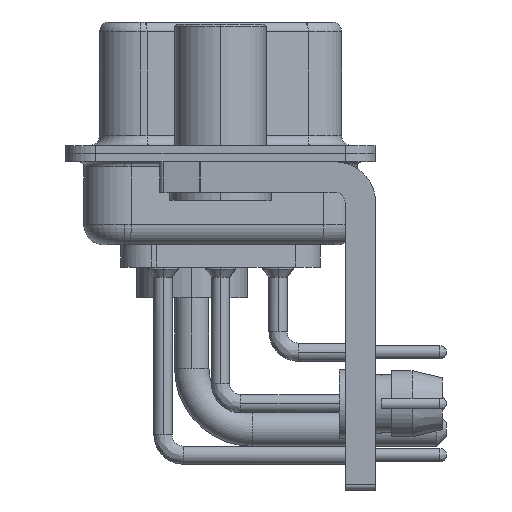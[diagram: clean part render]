
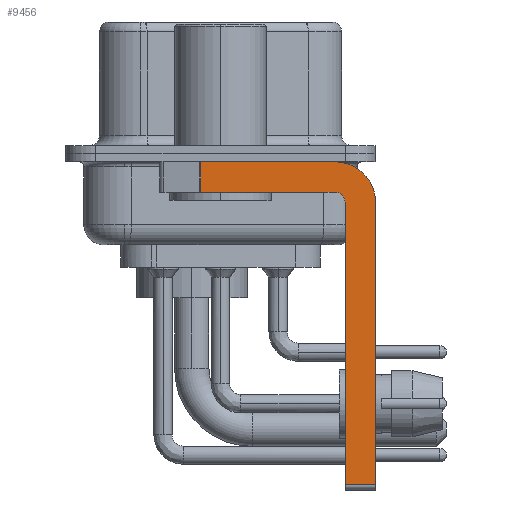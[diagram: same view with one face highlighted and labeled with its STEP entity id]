
A CAD part, left-side view. The second image highlights one B-rep face of the part: STEP entity #9456.
In plain terms, the highlighted planar face has unit normal (-1, 0, 0).
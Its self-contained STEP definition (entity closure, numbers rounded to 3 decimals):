
#649 = LINE ( 'NONE', #10176, #8430 ) ;
#1288 = VECTOR ( 'NONE', #22207, 1000. ) ;
#1503 = CARTESIAN_POINT ( 'NONE',  ( -2.9, -5.65, -2.4 ) ) ;
#1557 = DIRECTION ( 'NONE',  ( 0., 1., 0. ) ) ;
#1679 = CARTESIAN_POINT ( 'NONE',  ( -2.9, -5.65, -0.4 ) ) ;
#4796 = CARTESIAN_POINT ( 'NONE',  ( -2.9, -5.65, -2.4 ) ) ;
#5149 = ORIENTED_EDGE ( 'NONE', *, *, #18182, .T. ) ;
#5592 = EDGE_CURVE ( 'NONE', #38702, #24365, #30042, .T. ) ;
#5847 = CARTESIAN_POINT ( 'NONE',  ( -2.9, 0.978, -0.4 ) ) ;
#6621 = CARTESIAN_POINT ( 'NONE',  ( -2.9, -5.65, -2.4 ) ) ;
#6799 = DIRECTION ( 'NONE',  ( 0., -1., 0. ) ) ;
#8084 = DIRECTION ( 'NONE',  ( 0., -1., 0. ) ) ;
#8430 = VECTOR ( 'NONE', #22807, 1000. ) ;
#9301 = VERTEX_POINT ( 'NONE', #25941 ) ;
#9351 = VERTEX_POINT ( 'NONE', #12679 ) ;
#9456 = ADVANCED_FACE ( 'NONE', ( #14325 ), #29455, .F. ) ;
#9795 = AXIS2_PLACEMENT_3D ( 'NONE', #6621, #37888, #15529 ) ;
#10176 = CARTESIAN_POINT ( 'NONE',  ( -2.9, -7.65, -2.4 ) ) ;
#10959 = ORIENTED_EDGE ( 'NONE', *, *, #39089, .F. ) ;
#11698 = VECTOR ( 'NONE', #1557, 1000. ) ;
#12417 = ORIENTED_EDGE ( 'NONE', *, *, #38872, .T. ) ;
#12679 = CARTESIAN_POINT ( 'NONE',  ( -2.9, -6.15, -2.4 ) ) ;
#12680 = CARTESIAN_POINT ( 'NONE',  ( -2.9, 0.978, -1.9 ) ) ;
#12771 = AXIS2_PLACEMENT_3D ( 'NONE', #1503, #17257, #29246 ) ;
#14325 = FACE_OUTER_BOUND ( 'NONE', #33681, .T. ) ;
#15198 = AXIS2_PLACEMENT_3D ( 'NONE', #4796, #23451, #36061 ) ;
#15529 = DIRECTION ( 'NONE',  ( 0., 0., 1. ) ) ;
#16122 = LINE ( 'NONE', #28753, #18480 ) ;
#16672 = CARTESIAN_POINT ( 'NONE',  ( -2.9, -5.65, -1.9 ) ) ;
#17257 = DIRECTION ( 'NONE',  ( 1., 0., 0. ) ) ;
#17789 = ORIENTED_EDGE ( 'NONE', *, *, #5592, .F. ) ;
#18182 = EDGE_CURVE ( 'NONE', #24599, #9301, #16122, .T. ) ;
#18466 = CARTESIAN_POINT ( 'NONE',  ( -2.9, -6.15, -16.6 ) ) ;
#18480 = VECTOR ( 'NONE', #6799, 1000. ) ;
#19978 = LINE ( 'NONE', #16672, #11698 ) ;
#20207 = EDGE_CURVE ( 'NONE', #28423, #9301, #649, .T. ) ;
#20610 = EDGE_CURVE ( 'NONE', #9351, #23227, #26328, .T. ) ;
#21764 = LINE ( 'NONE', #18466, #39908 ) ;
#22207 = DIRECTION ( 'NONE',  ( 0., 0., -1. ) ) ;
#22807 = DIRECTION ( 'NONE',  ( 0., 0., -1. ) ) ;
#23227 = VERTEX_POINT ( 'NONE', #28762 ) ;
#23451 = DIRECTION ( 'NONE',  ( 1., 0., 0. ) ) ;
#24365 = VERTEX_POINT ( 'NONE', #1679 ) ;
#24599 = VERTEX_POINT ( 'NONE', #40765 ) ;
#25451 = ORIENTED_EDGE ( 'NONE', *, *, #35139, .F. ) ;
#25941 = CARTESIAN_POINT ( 'NONE',  ( -2.9, -7.65, -16.35 ) ) ;
#26328 = CIRCLE ( 'NONE', #9795, 0.5 ) ;
#27676 = ORIENTED_EDGE ( 'NONE', *, *, #20610, .F. ) ;
#28423 = VERTEX_POINT ( 'NONE', #40656 ) ;
#28437 = LINE ( 'NONE', #12680, #1288 ) ;
#28753 = CARTESIAN_POINT ( 'NONE',  ( -2.9, -5.65, -16.35 ) ) ;
#28762 = CARTESIAN_POINT ( 'NONE',  ( -2.9, -5.65, -1.9 ) ) ;
#29246 = DIRECTION ( 'NONE',  ( 0., 0., -1. ) ) ;
#29455 = PLANE ( 'NONE',  #12771 ) ;
#30042 = LINE ( 'NONE', #36444, #33720 ) ;
#31657 = EDGE_CURVE ( 'NONE', #24599, #9351, #21764, .T. ) ;
#33681 = EDGE_LOOP ( 'NONE', ( #17789, #12417, #25451, #27676, #38860, #5149, #40332, #10959 ) ) ;
#33720 = VECTOR ( 'NONE', #8084, 1000. ) ;
#35139 = EDGE_CURVE ( 'NONE', #23227, #40680, #19978, .T. ) ;
#36061 = DIRECTION ( 'NONE',  ( 0., 0., -1. ) ) ;
#36444 = CARTESIAN_POINT ( 'NONE',  ( -2.9, 3., -0.4 ) ) ;
#37009 = CIRCLE ( 'NONE', #15198, 2. ) ;
#37888 = DIRECTION ( 'NONE',  ( -1., 0., 0. ) ) ;
#37904 = CARTESIAN_POINT ( 'NONE',  ( -2.9, 0.978, -1.9 ) ) ;
#38702 = VERTEX_POINT ( 'NONE', #5847 ) ;
#38860 = ORIENTED_EDGE ( 'NONE', *, *, #31657, .F. ) ;
#38872 = EDGE_CURVE ( 'NONE', #38702, #40680, #28437, .T. ) ;
#39089 = EDGE_CURVE ( 'NONE', #24365, #28423, #37009, .T. ) ;
#39908 = VECTOR ( 'NONE', #40196, 1000. ) ;
#40196 = DIRECTION ( 'NONE',  ( 0., 0., 1. ) ) ;
#40332 = ORIENTED_EDGE ( 'NONE', *, *, #20207, .F. ) ;
#40656 = CARTESIAN_POINT ( 'NONE',  ( -2.9, -7.65, -2.4 ) ) ;
#40680 = VERTEX_POINT ( 'NONE', #37904 ) ;
#40765 = CARTESIAN_POINT ( 'NONE',  ( -2.9, -6.15, -16.35 ) ) ;
